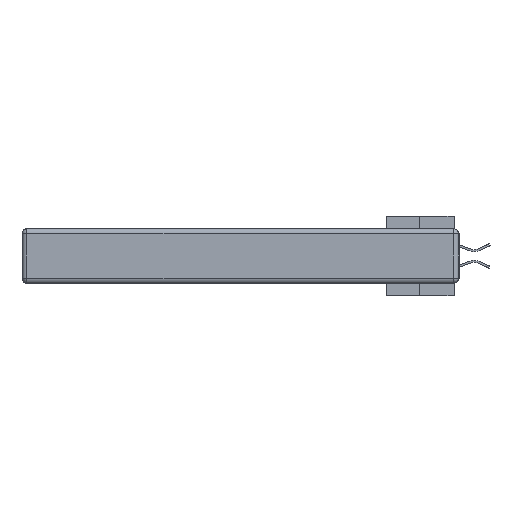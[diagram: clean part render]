
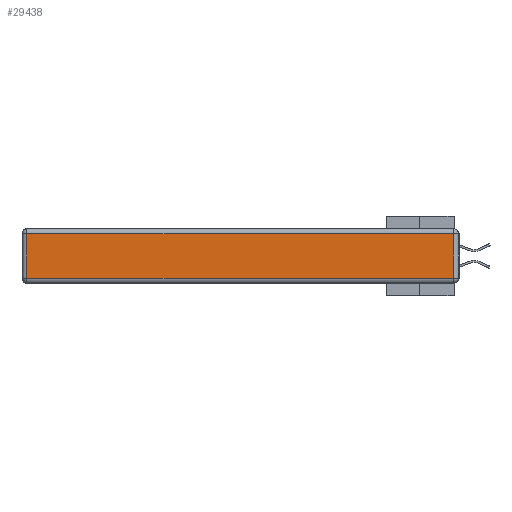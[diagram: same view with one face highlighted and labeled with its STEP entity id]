
A CAD part, left-side view. The second image highlights one B-rep face of the part: STEP entity #29438.
In plain terms, the highlighted planar face has unit normal (-1, 0, 0).
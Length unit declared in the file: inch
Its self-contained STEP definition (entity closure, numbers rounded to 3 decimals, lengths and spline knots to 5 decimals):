
#44 = CARTESIAN_POINT ( 'NONE',  ( 0., 2.72, -0.313 ) ) ;
#723 = VERTEX_POINT ( 'NONE', #16784 ) ;
#2056 = EDGE_LOOP ( 'NONE', ( #37950, #14904, #7311, #7219 ) ) ;
#3299 = DIRECTION ( 'NONE',  ( 0., 1., 0. ) ) ;
#3974 = VECTOR ( 'NONE', #22049, 39.37008 ) ;
#5033 = PLANE ( 'NONE',  #33091 ) ;
#6289 = LINE ( 'NONE', #15142, #26994 ) ;
#7219 = ORIENTED_EDGE ( 'NONE', *, *, #14714, .T. ) ;
#7311 = ORIENTED_EDGE ( 'NONE', *, *, #37066, .T. ) ;
#8024 = DIRECTION ( 'NONE',  ( -1., 0., 0. ) ) ;
#8657 = LINE ( 'NONE', #9473, #12990 ) ;
#8878 = VECTOR ( 'NONE', #28779, 39.37008 ) ;
#9473 = CARTESIAN_POINT ( 'NONE',  ( 0., 2.75, -0.03 ) ) ;
#12006 = DIRECTION ( 'NONE',  ( 0., 0., -1. ) ) ;
#12873 = EDGE_CURVE ( 'NONE', #18868, #723, #34769, .T. ) ;
#12990 = VECTOR ( 'NONE', #3299, 39.37008 ) ;
#14714 = EDGE_CURVE ( 'NONE', #31764, #18868, #6289, .T. ) ;
#14904 = ORIENTED_EDGE ( 'NONE', *, *, #33659, .T. ) ;
#15142 = CARTESIAN_POINT ( 'NONE',  ( 0., 2.72, -0.343 ) ) ;
#16570 = FACE_OUTER_BOUND ( 'NONE', #2056, .T. ) ;
#16784 = CARTESIAN_POINT ( 'NONE',  ( 0., 0.03, -0.313 ) ) ;
#17711 = CARTESIAN_POINT ( 'NONE',  ( 0., 0., -0.343 ) ) ;
#18868 = VERTEX_POINT ( 'NONE', #44 ) ;
#19984 = LINE ( 'NONE', #28651, #8878 ) ;
#20237 = DIRECTION ( 'NONE',  ( 0., 0., 1. ) ) ;
#21511 = CARTESIAN_POINT ( 'NONE',  ( 0., 0., -0.313 ) ) ;
#22049 = DIRECTION ( 'NONE',  ( 0., -1., 0. ) ) ;
#24496 = CARTESIAN_POINT ( 'NONE',  ( 0., 2.72, -0.03 ) ) ;
#24631 = CARTESIAN_POINT ( 'NONE',  ( 0., 0.03, -0.03 ) ) ;
#26567 = VERTEX_POINT ( 'NONE', #24631 ) ;
#26994 = VECTOR ( 'NONE', #12006, 39.37008 ) ;
#28651 = CARTESIAN_POINT ( 'NONE',  ( 0., 0.03, -0.343 ) ) ;
#28779 = DIRECTION ( 'NONE',  ( 0., 0., 1. ) ) ;
#29438 = ADVANCED_FACE ( 'NONE', ( #16570 ), #5033, .T. ) ;
#31764 = VERTEX_POINT ( 'NONE', #24496 ) ;
#33091 = AXIS2_PLACEMENT_3D ( 'NONE', #17711, #8024, #20237 ) ;
#33659 = EDGE_CURVE ( 'NONE', #723, #26567, #19984, .T. ) ;
#34769 = LINE ( 'NONE', #21511, #3974 ) ;
#37066 = EDGE_CURVE ( 'NONE', #26567, #31764, #8657, .T. ) ;
#37950 = ORIENTED_EDGE ( 'NONE', *, *, #12873, .T. ) ;
